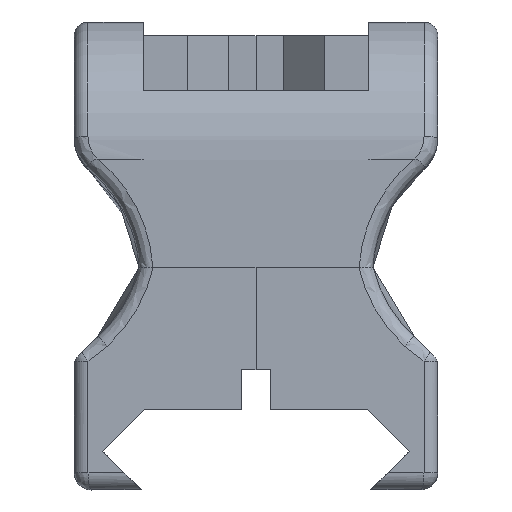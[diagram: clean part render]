
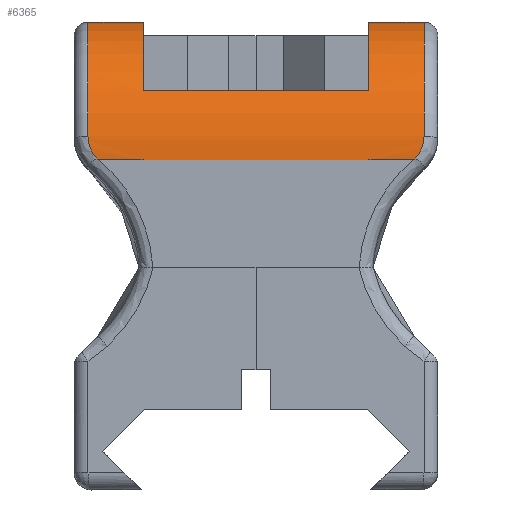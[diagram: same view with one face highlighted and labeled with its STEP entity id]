
A CAD part, front view. The second image highlights one B-rep face of the part: STEP entity #6365.
In plain terms, the highlighted cylindrical face has radius 10 mm (diameter 20 mm), a partial arc.
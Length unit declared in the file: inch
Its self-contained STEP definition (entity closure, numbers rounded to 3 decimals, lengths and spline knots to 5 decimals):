
#72=CYLINDRICAL_SURFACE('',#6823,0.3937);
#318=B_SPLINE_CURVE_WITH_KNOTS('',3,(#12173,#12174,#12175,#12176,#12177,
#12178,#12179),.UNSPECIFIED.,.F.,.F.,(4,3,4),(-0.00358,0.,0.00455),
 .UNSPECIFIED.);
#323=B_SPLINE_CURVE_WITH_KNOTS('',3,(#12269,#12270,#12271,#12272,#12273),
 .UNSPECIFIED.,.F.,.F.,(4,1,4),(-0.16965,-0.08483,
0.),.UNSPECIFIED.);
#324=B_SPLINE_CURVE_WITH_KNOTS('',3,(#12321,#12322,#12323,#12324,#12325,
#12326,#12327),.UNSPECIFIED.,.F.,.F.,(4,3,4),(-0.00358,0.,0.00455),
 .UNSPECIFIED.);
#325=B_SPLINE_CURVE_WITH_KNOTS('',3,(#12329,#12330,#12331,#12332,#12333),
 .UNSPECIFIED.,.F.,.F.,(4,1,4),(-0.16965,-0.08483,
0.),.UNSPECIFIED.);
#357=CIRCLE('',#6473,0.3937);
#386=CIRCLE('',#6537,0.3937);
#462=CIRCLE('',#6818,0.3937);
#464=CIRCLE('',#6824,0.3937);
#465=CIRCLE('',#6825,0.3937);
#466=CIRCLE('',#6826,0.3937);
#821=FACE_OUTER_BOUND('',#1170,.T.);
#1170=EDGE_LOOP('',(#5540,#5541,#5542,#5543,#5544,#5545,#5546,#5547,#5548,
#5549,#5550,#5551,#5552,#5553,#5554,#5555));
#1616=LINE('',#11418,#2196);
#1719=LINE('',#12242,#2299);
#1725=LINE('',#12311,#2305);
#1726=LINE('',#12315,#2306);
#1727=LINE('',#12319,#2307);
#1728=LINE('',#12336,#2308);
#2196=VECTOR('',#7871,0.3937);
#2299=VECTOR('',#8138,0.3937);
#2305=VECTOR('',#8160,0.3937);
#2306=VECTOR('',#8163,0.3937);
#2307=VECTOR('',#8166,0.3937);
#2308=VECTOR('',#8169,0.3937);
#2489=VERTEX_POINT('',#8670);
#2490=VERTEX_POINT('',#8672);
#2609=VERTEX_POINT('',#9459);
#2611=VERTEX_POINT('',#9462);
#2920=VERTEX_POINT('',#12105);
#2922=VERTEX_POINT('',#12165);
#2925=VERTEX_POINT('',#12238);
#2926=VERTEX_POINT('',#12268);
#2930=VERTEX_POINT('',#12310);
#2931=VERTEX_POINT('',#12312);
#2932=VERTEX_POINT('',#12314);
#2933=VERTEX_POINT('',#12316);
#2934=VERTEX_POINT('',#12318);
#2935=VERTEX_POINT('',#12320);
#2936=VERTEX_POINT('',#12328);
#2937=VERTEX_POINT('',#12334);
#3114=EDGE_CURVE('',#2490,#2489,#357,.T.);
#3271=EDGE_CURVE('',#2609,#2611,#386,.T.);
#3653=EDGE_CURVE('',#2490,#2609,#1616,.T.);
#3812=EDGE_CURVE('',#2922,#2920,#318,.T.);
#3820=EDGE_CURVE('',#2925,#2489,#1719,.T.);
#3821=EDGE_CURVE('',#2920,#2926,#323,.T.);
#3823=EDGE_CURVE('',#2926,#2925,#462,.T.);
#3830=EDGE_CURVE('',#2930,#2922,#1725,.T.);
#3831=EDGE_CURVE('',#2930,#2931,#464,.T.);
#3832=EDGE_CURVE('',#2932,#2931,#1726,.T.);
#3833=EDGE_CURVE('',#2933,#2932,#465,.T.);
#3834=EDGE_CURVE('',#2933,#2934,#1727,.T.);
#3835=EDGE_CURVE('',#2934,#2935,#324,.T.);
#3836=EDGE_CURVE('',#2935,#2936,#325,.T.);
#3837=EDGE_CURVE('',#2936,#2937,#466,.T.);
#3838=EDGE_CURVE('',#2937,#2611,#1728,.T.);
#5540=ORIENTED_EDGE('',*,*,#3653,.F.);
#5541=ORIENTED_EDGE('',*,*,#3114,.T.);
#5542=ORIENTED_EDGE('',*,*,#3820,.F.);
#5543=ORIENTED_EDGE('',*,*,#3823,.F.);
#5544=ORIENTED_EDGE('',*,*,#3821,.F.);
#5545=ORIENTED_EDGE('',*,*,#3812,.F.);
#5546=ORIENTED_EDGE('',*,*,#3830,.F.);
#5547=ORIENTED_EDGE('',*,*,#3831,.T.);
#5548=ORIENTED_EDGE('',*,*,#3832,.F.);
#5549=ORIENTED_EDGE('',*,*,#3833,.F.);
#5550=ORIENTED_EDGE('',*,*,#3834,.T.);
#5551=ORIENTED_EDGE('',*,*,#3835,.T.);
#5552=ORIENTED_EDGE('',*,*,#3836,.T.);
#5553=ORIENTED_EDGE('',*,*,#3837,.T.);
#5554=ORIENTED_EDGE('',*,*,#3838,.T.);
#5555=ORIENTED_EDGE('',*,*,#3271,.F.);
#6365=ADVANCED_FACE('',(#821),#72,.T.);
#6473=AXIS2_PLACEMENT_3D('',#8673,#7047,#7048);
#6537=AXIS2_PLACEMENT_3D('',#9463,#7253,#7254);
#6818=AXIS2_PLACEMENT_3D('',#12276,#8143,#8144);
#6823=AXIS2_PLACEMENT_3D('',#12309,#8158,#8159);
#6824=AXIS2_PLACEMENT_3D('',#12313,#8161,#8162);
#6825=AXIS2_PLACEMENT_3D('',#12317,#8164,#8165);
#6826=AXIS2_PLACEMENT_3D('',#12335,#8167,#8168);
#7047=DIRECTION('center_axis',(-1.,0.,0.));
#7048=DIRECTION('ref_axis',(0.,0.707,0.707));
#7253=DIRECTION('center_axis',(-1.,0.,
0.));
#7254=DIRECTION('ref_axis',(0.,0.707,0.707));
#7871=DIRECTION('',(1.,0.,0.));
#8138=DIRECTION('',(1.,0.,0.));
#8143=DIRECTION('center_axis',(-1.,0.,
0.));
#8144=DIRECTION('ref_axis',(0.,-0.804,0.595));
#8158=DIRECTION('center_axis',(-1.,0.,
0.));
#8159=DIRECTION('ref_axis',(0.,-0.707,0.707));
#8160=DIRECTION('',(-1.,0.,0.));
#8161=DIRECTION('center_axis',(1.,0.,0.));
#8162=DIRECTION('ref_axis',(0.,-0.707,0.707));
#8163=DIRECTION('',(-1.,0.,0.));
#8164=DIRECTION('center_axis',(1.,0.,0.));
#8165=DIRECTION('ref_axis',(0.,-0.707,0.707));
#8166=DIRECTION('',(1.,0.,0.));
#8167=DIRECTION('center_axis',(-1.,0.,
0.));
#8168=DIRECTION('ref_axis',(0.,-0.804,0.595));
#8169=DIRECTION('',(-1.,0.,0.));
#8670=CARTESIAN_POINT('',(-0.32791,-8.53604,1.0995));
#8672=CARTESIAN_POINT('',(-0.32791,-8.8745,0.90265));
#8673=CARTESIAN_POINT('Origin',(-0.32791,-8.53354,0.7058));
#9459=CARTESIAN_POINT('',(0.31863,-8.8745,0.90265));
#9462=CARTESIAN_POINT('',(0.31863,-8.53604,1.0995));
#9463=CARTESIAN_POINT('Origin',(0.31863,-8.53354,0.7058));
#11418=CARTESIAN_POINT('',(-0.16627,-8.8745,0.90265));
#12105=CARTESIAN_POINT('',(-0.45893,-8.92724,0.70741));
#12165=CARTESIAN_POINT('',(-0.45616,-8.92724,0.7058));
#12173=CARTESIAN_POINT('Ctrl Pts',(-0.45616,-8.92724,
0.7058));
#12174=CARTESIAN_POINT('Ctrl Pts',(-0.45657,-8.92724,
0.70604));
#12175=CARTESIAN_POINT('Ctrl Pts',(-0.45697,-8.92724,
0.70627));
#12176=CARTESIAN_POINT('Ctrl Pts',(-0.45738,-8.92724,
0.70651));
#12177=CARTESIAN_POINT('Ctrl Pts',(-0.45789,-8.92724,
0.70681));
#12178=CARTESIAN_POINT('Ctrl Pts',(-0.45841,-8.92724,
0.70711));
#12179=CARTESIAN_POINT('Ctrl Pts',(-0.45893,-8.92724,
0.70741));
#12238=CARTESIAN_POINT('',(-0.48539,-8.53604,1.0995));
#12242=CARTESIAN_POINT('',(0.157,-8.53604,1.0995));
#12268=CARTESIAN_POINT('',(-0.48539,-8.92149,0.77283));
#12269=CARTESIAN_POINT('Ctrl Pts',(-0.45893,-8.92724,
0.70741));
#12270=CARTESIAN_POINT('Ctrl Pts',(-0.46725,-8.92721,
0.71563));
#12271=CARTESIAN_POINT('Ctrl Pts',(-0.48071,-8.92659,
0.73605));
#12272=CARTESIAN_POINT('Ctrl Pts',(-0.48539,-8.9236,
0.76065));
#12273=CARTESIAN_POINT('Ctrl Pts',(-0.48539,-8.92149,0.77283));
#12276=CARTESIAN_POINT('Origin',(-0.48539,-8.53354,0.7058));
#12309=CARTESIAN_POINT('Origin',(0.157,-8.53354,0.7058));
#12310=CARTESIAN_POINT('',(-0.32791,-8.92724,0.7058));
#12311=CARTESIAN_POINT('',(-0.32791,-8.92724,0.7058));
#12312=CARTESIAN_POINT('',(-0.32791,-8.92724,0.7058));
#12313=CARTESIAN_POINT('Origin',(-0.32791,-8.53354,0.7058));
#12314=CARTESIAN_POINT('',(0.31863,-8.92724,0.7058));
#12315=CARTESIAN_POINT('',(-0.16627,-8.92724,0.7058));
#12316=CARTESIAN_POINT('',(0.31863,-8.92724,0.7058));
#12317=CARTESIAN_POINT('Origin',(0.31863,-8.53354,0.7058));
#12318=CARTESIAN_POINT('',(0.44689,-8.92724,0.7058));
#12319=CARTESIAN_POINT('',(0.31863,-8.92724,0.7058));
#12320=CARTESIAN_POINT('',(0.44966,-8.92724,0.70741));
#12321=CARTESIAN_POINT('Ctrl Pts',(0.44689,-8.92724,
0.7058));
#12322=CARTESIAN_POINT('Ctrl Pts',(0.4473,-8.92724,
0.70604));
#12323=CARTESIAN_POINT('Ctrl Pts',(0.4477,-8.92724,0.70627));
#12324=CARTESIAN_POINT('Ctrl Pts',(0.44811,-8.92724,0.70651));
#12325=CARTESIAN_POINT('Ctrl Pts',(0.44862,-8.92724,
0.70681));
#12326=CARTESIAN_POINT('Ctrl Pts',(0.44914,-8.92724,
0.70711));
#12327=CARTESIAN_POINT('Ctrl Pts',(0.44966,-8.92724,
0.70741));
#12328=CARTESIAN_POINT('',(0.47611,-8.92149,0.77283));
#12329=CARTESIAN_POINT('Ctrl Pts',(0.44966,-8.92724,
0.70741));
#12330=CARTESIAN_POINT('Ctrl Pts',(0.45798,-8.92721,0.71563));
#12331=CARTESIAN_POINT('Ctrl Pts',(0.47144,-8.92659,
0.73605));
#12332=CARTESIAN_POINT('Ctrl Pts',(0.47611,-8.9236,
0.76065));
#12333=CARTESIAN_POINT('Ctrl Pts',(0.47611,-8.92149,
0.77283));
#12334=CARTESIAN_POINT('',(0.47611,-8.53604,1.0995));
#12335=CARTESIAN_POINT('Origin',(0.47611,-8.53354,0.7058));
#12336=CARTESIAN_POINT('',(-0.16627,-8.53604,1.0995));
